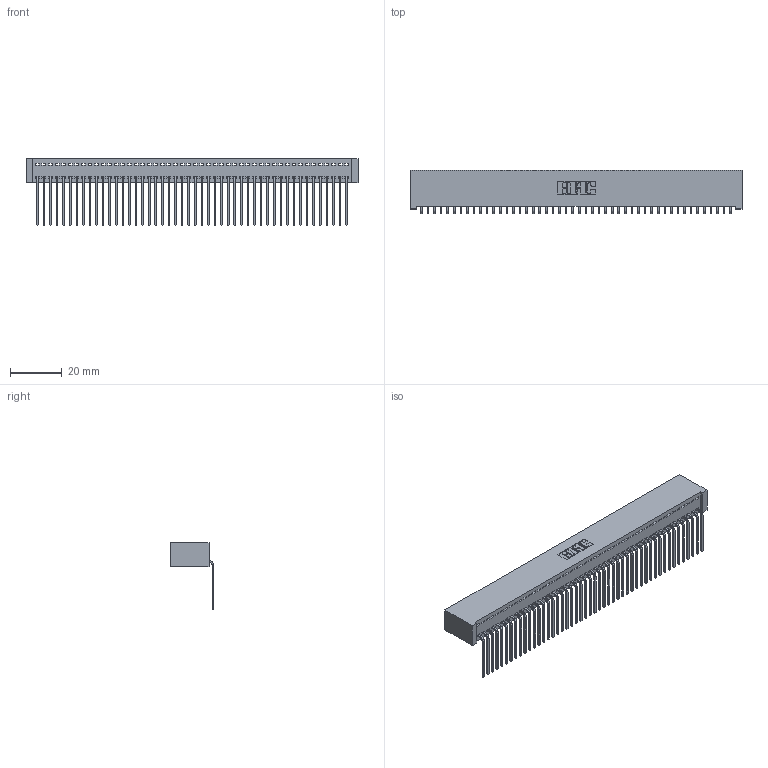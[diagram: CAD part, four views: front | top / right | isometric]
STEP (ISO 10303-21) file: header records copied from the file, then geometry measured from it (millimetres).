
FILE_DESCRIPTION (( 'STEP AP203' ), '1' );
FILE_NAME ('392-048-559-101.STEP', '2018-08-16T23:27:07', ( '' ), ( '' ), 'SwSTEP 2.0', 'SolidWorks 2016', '' );
FILE_SCHEMA (( 'CONFIG_CONTROL_DESIGN' ));
Length unit declared in the file: inch
Products named in the file (3): 342 Part_Lugless; 345-292-001_558 559 Tail - 1; 392-048-559-101
Assembly tree (49 placements, depth 2):
  392-048-559-101
    342 Part_Lugless
    345-292-001_558 559 Tail - 1  x48
Bounding box: 128.17 x 16.83 x 25.78 mm (x, y, z)
Volume: 11828.8 mm3; surface area: 18713.6 mm2
Topology: 49 solids, 49 shells, 2982 faces, 9011 edges, 5942 vertices
Faces by surface type: plane 2174, cylinder 808
Entity records: 28243 total; most frequent: CARTESIAN_POINT 4878, ORIENTED_EDGE 4862, DIRECTION 4095, EDGE_CURVE 2431, LINE 2311, VECTOR 2311, VERTEX_POINT 1618, AXIS2_PLACEMENT_3D 892
